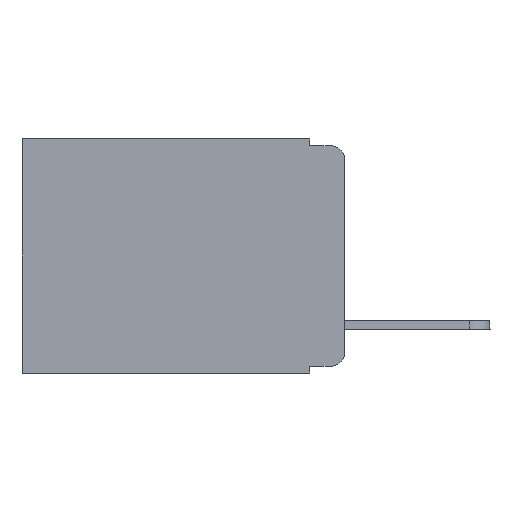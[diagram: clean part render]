
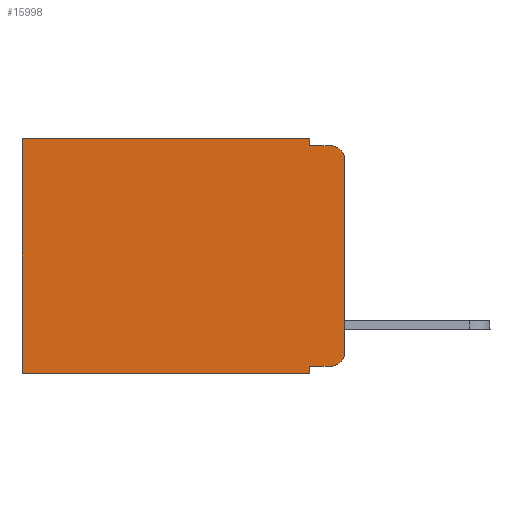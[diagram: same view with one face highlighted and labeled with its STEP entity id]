
A CAD part, left-side view. The second image highlights one B-rep face of the part: STEP entity #15998.
In plain terms, the highlighted planar face has unit normal (-1, 0, 0).
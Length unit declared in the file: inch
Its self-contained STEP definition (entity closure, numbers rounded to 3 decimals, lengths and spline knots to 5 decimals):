
#45 = DIRECTION ( 'NONE',  ( 0., 0., -1. ) ) ;
#692 = EDGE_CURVE ( 'NONE', #6378, #10191, #13230, .T. ) ;
#890 = DIRECTION ( 'NONE',  ( 0., 0., -1. ) ) ;
#1062 = CARTESIAN_POINT ( 'NONE',  ( 0.298, 0., 0. ) ) ;
#1171 = VECTOR ( 'NONE', #18431, 39.37008 ) ;
#1238 = ORIENTED_EDGE ( 'NONE', *, *, #1367, .T. ) ;
#1251 = EDGE_CURVE ( 'NONE', #10514, #9673, #1548, .T. ) ;
#1367 = EDGE_CURVE ( 'NONE', #11812, #10514, #12296, .T. ) ;
#1548 = CIRCLE ( 'NONE', #9638, 0.02 ) ;
#1725 = CARTESIAN_POINT ( 'NONE',  ( 0.298, 0., 0. ) ) ;
#2318 = DIRECTION ( 'NONE',  ( 0., 1., 0. ) ) ;
#2500 = CARTESIAN_POINT ( 'NONE',  ( 0.298, 0.02, -0.01 ) ) ;
#2632 = ORIENTED_EDGE ( 'NONE', *, *, #18115, .F. ) ;
#2807 = VECTOR ( 'NONE', #19668, 39.37008 ) ;
#2886 = EDGE_CURVE ( 'NONE', #3202, #16821, #19412, .T. ) ;
#2960 = DIRECTION ( 'NONE',  ( 0., 1., 0. ) ) ;
#3076 = CARTESIAN_POINT ( 'NONE',  ( 0.298, 0.051, -0.343 ) ) ;
#3202 = VERTEX_POINT ( 'NONE', #10552 ) ;
#3494 = CARTESIAN_POINT ( 'NONE',  ( 0.298, 0.473, 0. ) ) ;
#3534 = CARTESIAN_POINT ( 'NONE',  ( 0.298, 0.051, -0.333 ) ) ;
#3588 = CARTESIAN_POINT ( 'NONE',  ( 0.298, 0., 0. ) ) ;
#3900 = CARTESIAN_POINT ( 'NONE',  ( 0.298, 0.051, -0.333 ) ) ;
#3968 = CARTESIAN_POINT ( 'NONE',  ( 0.298, 0., -0.343 ) ) ;
#4807 = EDGE_CURVE ( 'NONE', #18246, #16821, #7959, .T. ) ;
#5570 = ORIENTED_EDGE ( 'NONE', *, *, #10680, .T. ) ;
#5994 = VECTOR ( 'NONE', #2318, 39.37008 ) ;
#6024 = CARTESIAN_POINT ( 'NONE',  ( 0.298, 0., -0.313 ) ) ;
#6378 = VERTEX_POINT ( 'NONE', #10843 ) ;
#7220 = ORIENTED_EDGE ( 'NONE', *, *, #1251, .T. ) ;
#7959 = CIRCLE ( 'NONE', #10097, 0.02 ) ;
#7984 = VERTEX_POINT ( 'NONE', #14776 ) ;
#8578 = DIRECTION ( 'NONE',  ( 0., 0., -1. ) ) ;
#8792 = ORIENTED_EDGE ( 'NONE', *, *, #692, .T. ) ;
#8892 = DIRECTION ( 'NONE',  ( 0., -1., 0. ) ) ;
#9129 = CARTESIAN_POINT ( 'NONE',  ( 0.298, 0.051, -0.01 ) ) ;
#9638 = AXIS2_PLACEMENT_3D ( 'NONE', #15213, #10328, #45 ) ;
#9673 = VERTEX_POINT ( 'NONE', #6024 ) ;
#9874 = DIRECTION ( 'NONE',  ( -1., 0., 0. ) ) ;
#10097 = AXIS2_PLACEMENT_3D ( 'NONE', #19932, #9874, #14956 ) ;
#10174 = CARTESIAN_POINT ( 'NONE',  ( 0.298, 0.473, 0. ) ) ;
#10191 = VERTEX_POINT ( 'NONE', #10174 ) ;
#10328 = DIRECTION ( 'NONE',  ( -1., 0., 0. ) ) ;
#10336 = DIRECTION ( 'NONE',  ( 0., 0., -1. ) ) ;
#10514 = VERTEX_POINT ( 'NONE', #16016 ) ;
#10552 = CARTESIAN_POINT ( 'NONE',  ( 0.298, 0.051, -0.01 ) ) ;
#10559 = DIRECTION ( 'NONE',  ( 1., 0., 0. ) ) ;
#10680 = EDGE_CURVE ( 'NONE', #10191, #7984, #11894, .T. ) ;
#10843 = CARTESIAN_POINT ( 'NONE',  ( 0.298, 0.051, 0. ) ) ;
#11458 = VECTOR ( 'NONE', #8578, 39.37008 ) ;
#11812 = VERTEX_POINT ( 'NONE', #3534 ) ;
#11894 = LINE ( 'NONE', #3494, #1171 ) ;
#12198 = PLANE ( 'NONE',  #13691 ) ;
#12296 = LINE ( 'NONE', #3900, #14619 ) ;
#12359 = VECTOR ( 'NONE', #890, 39.37008 ) ;
#12521 = FACE_OUTER_BOUND ( 'NONE', #17804, .T. ) ;
#12572 = EDGE_CURVE ( 'NONE', #18246, #9673, #18649, .T. ) ;
#12721 = CARTESIAN_POINT ( 'NONE',  ( 0.298, 0.051, 0. ) ) ;
#13230 = LINE ( 'NONE', #1062, #19132 ) ;
#13691 = AXIS2_PLACEMENT_3D ( 'NONE', #3588, #10559, #10336 ) ;
#14162 = CARTESIAN_POINT ( 'NONE',  ( 0.298, 0.051, 0. ) ) ;
#14259 = LINE ( 'NONE', #14162, #2807 ) ;
#14619 = VECTOR ( 'NONE', #8892, 39.37008 ) ;
#14776 = CARTESIAN_POINT ( 'NONE',  ( 0.298, 0.473, -0.343 ) ) ;
#14956 = DIRECTION ( 'NONE',  ( 0., 0., -1. ) ) ;
#15208 = VERTEX_POINT ( 'NONE', #3076 ) ;
#15213 = CARTESIAN_POINT ( 'NONE',  ( 0.298, 0.02, -0.313 ) ) ;
#15607 = LINE ( 'NONE', #3968, #5994 ) ;
#15998 = ADVANCED_FACE ( 'NONE', ( #12521 ), #12198, .F. ) ;
#16016 = CARTESIAN_POINT ( 'NONE',  ( 0.298, 0.02, -0.333 ) ) ;
#16563 = ORIENTED_EDGE ( 'NONE', *, *, #2886, .F. ) ;
#16751 = ORIENTED_EDGE ( 'NONE', *, *, #12572, .F. ) ;
#16821 = VERTEX_POINT ( 'NONE', #2500 ) ;
#17804 = EDGE_LOOP ( 'NONE', ( #16751, #18105, #16563, #21045, #8792, #5570, #2632, #21607, #1238, #7220 ) ) ;
#18105 = ORIENTED_EDGE ( 'NONE', *, *, #4807, .T. ) ;
#18115 = EDGE_CURVE ( 'NONE', #15208, #7984, #15607, .T. ) ;
#18246 = VERTEX_POINT ( 'NONE', #20985 ) ;
#18318 = EDGE_CURVE ( 'NONE', #6378, #3202, #14259, .T. ) ;
#18431 = DIRECTION ( 'NONE',  ( 0., 0., -1. ) ) ;
#18649 = LINE ( 'NONE', #1725, #11458 ) ;
#19121 = EDGE_CURVE ( 'NONE', #11812, #15208, #21234, .T. ) ;
#19132 = VECTOR ( 'NONE', #2960, 39.37008 ) ;
#19412 = LINE ( 'NONE', #9129, #19697 ) ;
#19668 = DIRECTION ( 'NONE',  ( 0., 0., -1. ) ) ;
#19697 = VECTOR ( 'NONE', #19744, 39.37008 ) ;
#19744 = DIRECTION ( 'NONE',  ( 0., -1., 0. ) ) ;
#19932 = CARTESIAN_POINT ( 'NONE',  ( 0.298, 0.02, -0.03 ) ) ;
#20985 = CARTESIAN_POINT ( 'NONE',  ( 0.298, 0., -0.03 ) ) ;
#21045 = ORIENTED_EDGE ( 'NONE', *, *, #18318, .F. ) ;
#21234 = LINE ( 'NONE', #12721, #12359 ) ;
#21607 = ORIENTED_EDGE ( 'NONE', *, *, #19121, .F. ) ;
